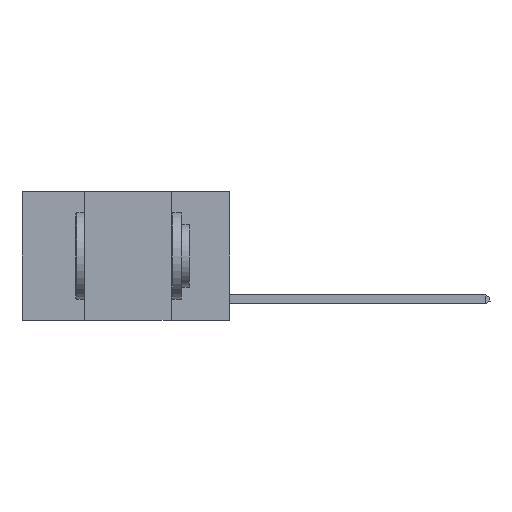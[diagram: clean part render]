
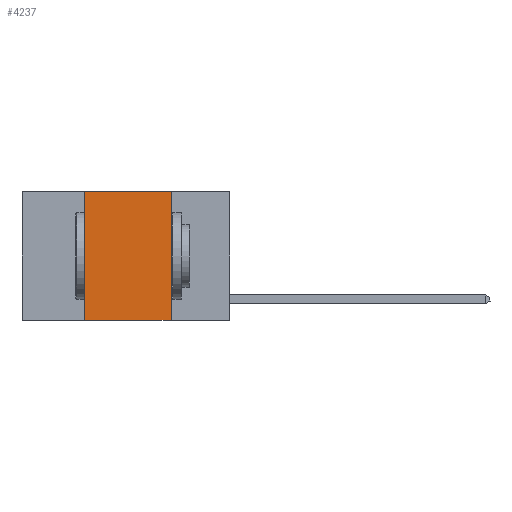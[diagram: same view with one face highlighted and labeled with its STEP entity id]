
A CAD part, left-side view. The second image highlights one B-rep face of the part: STEP entity #4237.
In plain terms, the highlighted planar face has unit normal (-1, 0, 0).
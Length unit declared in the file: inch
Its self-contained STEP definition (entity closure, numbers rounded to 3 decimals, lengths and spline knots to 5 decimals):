
#360 = VECTOR ( 'NONE', #18120, 39.37008 ) ;
#866 = CARTESIAN_POINT ( 'NONE',  ( 0., 0.6, 0. ) ) ;
#2630 = VERTEX_POINT ( 'NONE', #11987 ) ;
#3911 = PLANE ( 'NONE',  #9237 ) ;
#4237 = ADVANCED_FACE ( 'NONE', ( #23126 ), #3911, .F. ) ;
#5350 = LINE ( 'NONE', #14407, #360 ) ;
#5827 = DIRECTION ( 'NONE',  ( 1., 0., 0. ) ) ;
#8672 = VERTEX_POINT ( 'NONE', #20521 ) ;
#8989 = LINE ( 'NONE', #11143, #18276 ) ;
#9237 = AXIS2_PLACEMENT_3D ( 'NONE', #15118, #5827, #18805 ) ;
#9831 = VECTOR ( 'NONE', #17639, 39.37008 ) ;
#11143 = CARTESIAN_POINT ( 'NONE',  ( 0., 0.17, 0. ) ) ;
#11295 = VERTEX_POINT ( 'NONE', #19279 ) ;
#11987 = CARTESIAN_POINT ( 'NONE',  ( 0., 0.42, 0. ) ) ;
#13295 = VERTEX_POINT ( 'NONE', #17210 ) ;
#13793 = ORIENTED_EDGE ( 'NONE', *, *, #19528, .F. ) ;
#13928 = LINE ( 'NONE', #21662, #22500 ) ;
#14407 = CARTESIAN_POINT ( 'NONE',  ( 0., 0.6, -0.37 ) ) ;
#14805 = LINE ( 'NONE', #866, #9831 ) ;
#14939 = EDGE_CURVE ( 'NONE', #2630, #11295, #14805, .T. ) ;
#15118 = CARTESIAN_POINT ( 'NONE',  ( 0., 0.6, 0. ) ) ;
#16392 = ORIENTED_EDGE ( 'NONE', *, *, #19086, .F. ) ;
#17034 = EDGE_LOOP ( 'NONE', ( #16392, #21801, #13793, #18706 ) ) ;
#17068 = EDGE_CURVE ( 'NONE', #8672, #13295, #5350, .T. ) ;
#17210 = CARTESIAN_POINT ( 'NONE',  ( 0., 0.17, -0.37 ) ) ;
#17639 = DIRECTION ( 'NONE',  ( 0., -1., 0. ) ) ;
#18120 = DIRECTION ( 'NONE',  ( 0., -1., 0. ) ) ;
#18276 = VECTOR ( 'NONE', #18607, 39.37008 ) ;
#18607 = DIRECTION ( 'NONE',  ( 0., 0., -1. ) ) ;
#18706 = ORIENTED_EDGE ( 'NONE', *, *, #17068, .T. ) ;
#18805 = DIRECTION ( 'NONE',  ( 0., 0., -1. ) ) ;
#19086 = EDGE_CURVE ( 'NONE', #11295, #13295, #8989, .T. ) ;
#19279 = CARTESIAN_POINT ( 'NONE',  ( 0., 0.17, 0. ) ) ;
#19528 = EDGE_CURVE ( 'NONE', #8672, #2630, #13928, .T. ) ;
#20521 = CARTESIAN_POINT ( 'NONE',  ( 0., 0.42, -0.37 ) ) ;
#21662 = CARTESIAN_POINT ( 'NONE',  ( 0., 0.42, 0. ) ) ;
#21801 = ORIENTED_EDGE ( 'NONE', *, *, #14939, .F. ) ;
#22500 = VECTOR ( 'NONE', #23456, 39.37008 ) ;
#23126 = FACE_OUTER_BOUND ( 'NONE', #17034, .T. ) ;
#23456 = DIRECTION ( 'NONE',  ( 0., 0., 1. ) ) ;
